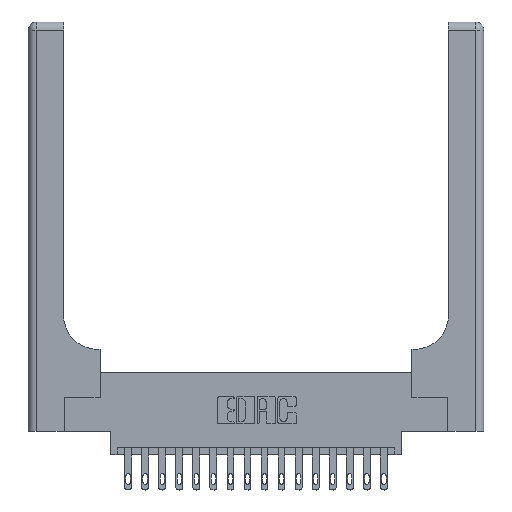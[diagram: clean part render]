
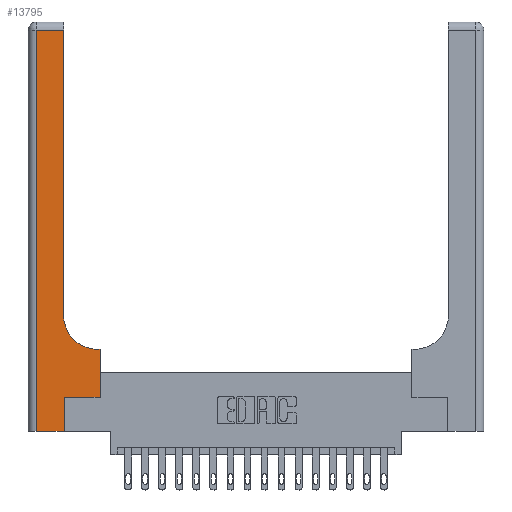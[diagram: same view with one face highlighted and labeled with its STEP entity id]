
A CAD part, top view. The second image highlights one B-rep face of the part: STEP entity #13795.
In plain terms, the highlighted planar face has unit normal (0, 0, 1).
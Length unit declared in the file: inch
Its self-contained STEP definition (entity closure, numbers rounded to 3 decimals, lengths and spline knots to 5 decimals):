
#238 = ORIENTED_EDGE ( 'NONE', *, *, #5301, .T. ) ;
#373 = AXIS2_PLACEMENT_3D ( 'NONE', #2137, #8184, #2240 ) ;
#379 = EDGE_CURVE ( 'NONE', #8626, #8575, #9740, .T. ) ;
#918 = ORIENTED_EDGE ( 'NONE', *, *, #3934, .T. ) ;
#1154 = LINE ( 'NONE', #8477, #11939 ) ;
#2137 = CARTESIAN_POINT ( 'NONE',  ( 0., 3., 0.37 ) ) ;
#2240 = DIRECTION ( 'NONE',  ( -1., 0., 0. ) ) ;
#2477 = CARTESIAN_POINT ( 'NONE',  ( 0.265, 0.25, 0.37 ) ) ;
#2596 = EDGE_CURVE ( 'NONE', #8575, #6599, #6930, .T. ) ;
#2862 = VECTOR ( 'NONE', #4459, 39.37008 ) ;
#3178 = EDGE_CURVE ( 'NONE', #3501, #3743, #1154, .T. ) ;
#3501 = VERTEX_POINT ( 'NONE', #16199 ) ;
#3503 = EDGE_LOOP ( 'NONE', ( #238, #13086, #11897, #5751, #6971, #918, #8711, #9540, #16739 ) ) ;
#3614 = EDGE_CURVE ( 'NONE', #3743, #3907, #10244, .T. ) ;
#3743 = VERTEX_POINT ( 'NONE', #5958 ) ;
#3754 = LINE ( 'NONE', #6625, #6491 ) ;
#3907 = VERTEX_POINT ( 'NONE', #17489 ) ;
#3934 = EDGE_CURVE ( 'NONE', #16314, #4979, #12986, .T. ) ;
#4411 = EDGE_CURVE ( 'NONE', #12770, #16314, #3754, .T. ) ;
#4459 = DIRECTION ( 'NONE',  ( 1., 0., 0. ) ) ;
#4898 = CARTESIAN_POINT ( 'NONE',  ( 0.528, 0.6, 0.37 ) ) ;
#4979 = VERTEX_POINT ( 'NONE', #7563 ) ;
#5119 = CARTESIAN_POINT ( 'NONE',  ( 0.51, 0.85, 0.37 ) ) ;
#5301 = EDGE_CURVE ( 'NONE', #6599, #3501, #17590, .T. ) ;
#5306 = FACE_OUTER_BOUND ( 'NONE', #3503, .T. ) ;
#5403 = DIRECTION ( 'NONE',  ( -1., 0., 0. ) ) ;
#5751 = ORIENTED_EDGE ( 'NONE', *, *, #18905, .T. ) ;
#5764 = CARTESIAN_POINT ( 'NONE',  ( 0.265, 0., 0.37 ) ) ;
#5958 = CARTESIAN_POINT ( 'NONE',  ( 0.06, 2.94, 0.37 ) ) ;
#6491 = VECTOR ( 'NONE', #17932, 39.37008 ) ;
#6571 = CARTESIAN_POINT ( 'NONE',  ( 0.26, 0.6, 0.37 ) ) ;
#6599 = VERTEX_POINT ( 'NONE', #9085 ) ;
#6625 = CARTESIAN_POINT ( 'NONE',  ( 0.265, 0., 0.37 ) ) ;
#6833 = VECTOR ( 'NONE', #16374, 39.37008 ) ;
#6930 = CIRCLE ( 'NONE', #16454, 0.25 ) ;
#6971 = ORIENTED_EDGE ( 'NONE', *, *, #4411, .T. ) ;
#6981 = VECTOR ( 'NONE', #18332, 39.37008 ) ;
#7429 = LINE ( 'NONE', #10787, #2862 ) ;
#7563 = CARTESIAN_POINT ( 'NONE',  ( 0.528, 0.25, 0.37 ) ) ;
#8184 = DIRECTION ( 'NONE',  ( 0., 0., -1. ) ) ;
#8477 = CARTESIAN_POINT ( 'NONE',  ( 0., 2.94, 0.37 ) ) ;
#8575 = VERTEX_POINT ( 'NONE', #18218 ) ;
#8626 = VERTEX_POINT ( 'NONE', #4898 ) ;
#8711 = ORIENTED_EDGE ( 'NONE', *, *, #12406, .T. ) ;
#9085 = CARTESIAN_POINT ( 'NONE',  ( 0.26, 0.85, 0.37 ) ) ;
#9277 = CARTESIAN_POINT ( 'NONE',  ( 0.528, 0.25, 0.37 ) ) ;
#9540 = ORIENTED_EDGE ( 'NONE', *, *, #379, .T. ) ;
#9664 = DIRECTION ( 'NONE',  ( 1., 0., 0. ) ) ;
#9740 = LINE ( 'NONE', #6571, #17804 ) ;
#10032 = DIRECTION ( 'NONE',  ( -1., 0., 0. ) ) ;
#10244 = LINE ( 'NONE', #16298, #17929 ) ;
#10769 = LINE ( 'NONE', #9277, #6981 ) ;
#10787 = CARTESIAN_POINT ( 'NONE',  ( 0., 0., 0.37 ) ) ;
#10926 = CARTESIAN_POINT ( 'NONE',  ( 0.265, 0.25, 0.37 ) ) ;
#11534 = DIRECTION ( 'NONE',  ( 0., 0., -1. ) ) ;
#11897 = ORIENTED_EDGE ( 'NONE', *, *, #3614, .T. ) ;
#11939 = VECTOR ( 'NONE', #5403, 39.37008 ) ;
#12406 = EDGE_CURVE ( 'NONE', #4979, #8626, #10769, .T. ) ;
#12770 = VERTEX_POINT ( 'NONE', #5764 ) ;
#12986 = LINE ( 'NONE', #2477, #17285 ) ;
#13086 = ORIENTED_EDGE ( 'NONE', *, *, #3178, .T. ) ;
#13795 = ADVANCED_FACE ( 'NONE', ( #5306 ), #15729, .F. ) ;
#14322 = DIRECTION ( 'NONE',  ( 0., -1., 0. ) ) ;
#15176 = CARTESIAN_POINT ( 'NONE',  ( 0.26, 3., 0.37 ) ) ;
#15729 = PLANE ( 'NONE',  #373 ) ;
#16199 = CARTESIAN_POINT ( 'NONE',  ( 0.26, 2.94, 0.37 ) ) ;
#16298 = CARTESIAN_POINT ( 'NONE',  ( 0.06, 3., 0.37 ) ) ;
#16314 = VERTEX_POINT ( 'NONE', #10926 ) ;
#16374 = DIRECTION ( 'NONE',  ( 0., 1., 0. ) ) ;
#16454 = AXIS2_PLACEMENT_3D ( 'NONE', #5119, #11534, #9664 ) ;
#16739 = ORIENTED_EDGE ( 'NONE', *, *, #2596, .T. ) ;
#17285 = VECTOR ( 'NONE', #18884, 39.37008 ) ;
#17489 = CARTESIAN_POINT ( 'NONE',  ( 0.06, 0., 0.37 ) ) ;
#17590 = LINE ( 'NONE', #15176, #6833 ) ;
#17804 = VECTOR ( 'NONE', #10032, 39.37008 ) ;
#17929 = VECTOR ( 'NONE', #14322, 39.37008 ) ;
#17932 = DIRECTION ( 'NONE',  ( 0., 1., 0. ) ) ;
#18218 = CARTESIAN_POINT ( 'NONE',  ( 0.51, 0.6, 0.37 ) ) ;
#18332 = DIRECTION ( 'NONE',  ( 0., 1., 0. ) ) ;
#18884 = DIRECTION ( 'NONE',  ( 1., 0., 0. ) ) ;
#18905 = EDGE_CURVE ( 'NONE', #3907, #12770, #7429, .T. ) ;
